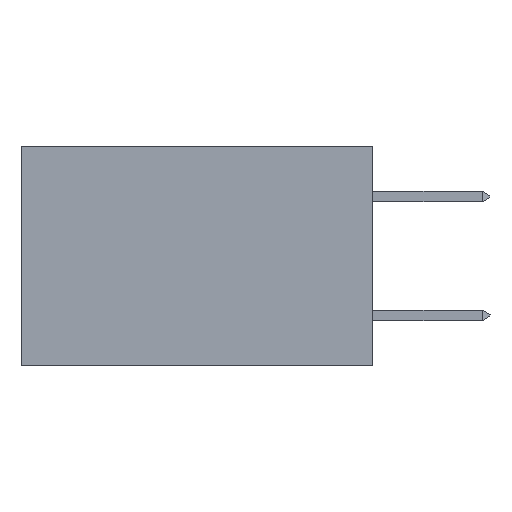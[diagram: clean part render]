
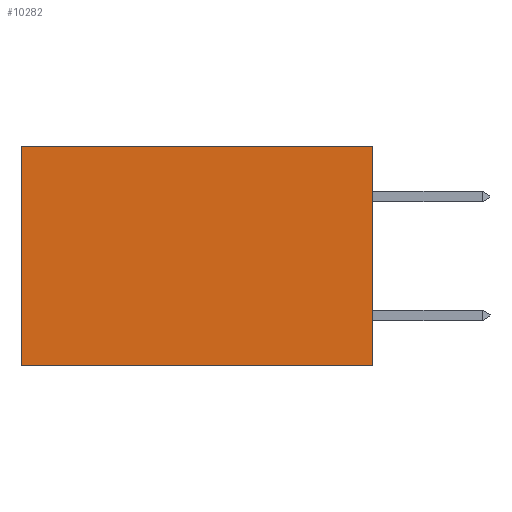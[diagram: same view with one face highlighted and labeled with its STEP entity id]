
A CAD part, left-side view. The second image highlights one B-rep face of the part: STEP entity #10282.
In plain terms, the highlighted planar face has unit normal (-1, 0, 0).
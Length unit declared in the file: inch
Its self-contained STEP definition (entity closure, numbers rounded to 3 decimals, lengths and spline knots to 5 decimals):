
#69 = LINE ( 'NONE', #908, #19425 ) ;
#908 = CARTESIAN_POINT ( 'NONE',  ( 0.277, 0., -0.37 ) ) ;
#1157 = LINE ( 'NONE', #6051, #5604 ) ;
#1227 = VERTEX_POINT ( 'NONE', #3277 ) ;
#1245 = EDGE_CURVE ( 'NONE', #9109, #1227, #69, .T. ) ;
#1263 = CARTESIAN_POINT ( 'NONE',  ( 0.277, 0.59, 0. ) ) ;
#1431 = ORIENTED_EDGE ( 'NONE', *, *, #7435, .T. ) ;
#1787 = CARTESIAN_POINT ( 'NONE',  ( 0.277, 0.59, -0.37 ) ) ;
#2344 = ORIENTED_EDGE ( 'NONE', *, *, #11164, .T. ) ;
#3277 = CARTESIAN_POINT ( 'NONE',  ( 0.277, 0., -0.37 ) ) ;
#5604 = VECTOR ( 'NONE', #5823, 39.37008 ) ;
#5823 = DIRECTION ( 'NONE',  ( 0., 0., -1. ) ) ;
#6051 = CARTESIAN_POINT ( 'NONE',  ( 0.277, 0.59, -0.37 ) ) ;
#7433 = DIRECTION ( 'NONE',  ( 0., 0., -1. ) ) ;
#7435 = EDGE_CURVE ( 'NONE', #18452, #12325, #1157, .T. ) ;
#7487 = DIRECTION ( 'NONE',  ( 1., 0., 0. ) ) ;
#7505 = CARTESIAN_POINT ( 'NONE',  ( 0.277, 0., -0.37 ) ) ;
#7825 = PLANE ( 'NONE',  #22480 ) ;
#9109 = VERTEX_POINT ( 'NONE', #21316 ) ;
#9390 = ORIENTED_EDGE ( 'NONE', *, *, #1245, .F. ) ;
#10033 = EDGE_CURVE ( 'NONE', #1227, #12325, #22634, .T. ) ;
#10239 = DIRECTION ( 'NONE',  ( 0., 1., 0. ) ) ;
#10282 = ADVANCED_FACE ( 'NONE', ( #17363 ), #7825, .F. ) ;
#10291 = CARTESIAN_POINT ( 'NONE',  ( 0.277, 0., -0.37 ) ) ;
#11164 = EDGE_CURVE ( 'NONE', #9109, #18452, #13819, .T. ) ;
#12267 = CARTESIAN_POINT ( 'NONE',  ( 0.277, 0., 0. ) ) ;
#12291 = DIRECTION ( 'NONE',  ( 0., 1., 0. ) ) ;
#12325 = VERTEX_POINT ( 'NONE', #1787 ) ;
#12814 = VECTOR ( 'NONE', #10239, 39.37008 ) ;
#13026 = ORIENTED_EDGE ( 'NONE', *, *, #10033, .F. ) ;
#13819 = LINE ( 'NONE', #12267, #14397 ) ;
#14397 = VECTOR ( 'NONE', #12291, 39.37008 ) ;
#16403 = EDGE_LOOP ( 'NONE', ( #1431, #13026, #9390, #2344 ) ) ;
#17363 = FACE_OUTER_BOUND ( 'NONE', #16403, .T. ) ;
#18452 = VERTEX_POINT ( 'NONE', #1263 ) ;
#19425 = VECTOR ( 'NONE', #21302, 39.37008 ) ;
#21302 = DIRECTION ( 'NONE',  ( 0., 0., -1. ) ) ;
#21316 = CARTESIAN_POINT ( 'NONE',  ( 0.277, 0., 0. ) ) ;
#22480 = AXIS2_PLACEMENT_3D ( 'NONE', #7505, #7487, #7433 ) ;
#22634 = LINE ( 'NONE', #10291, #12814 ) ;
